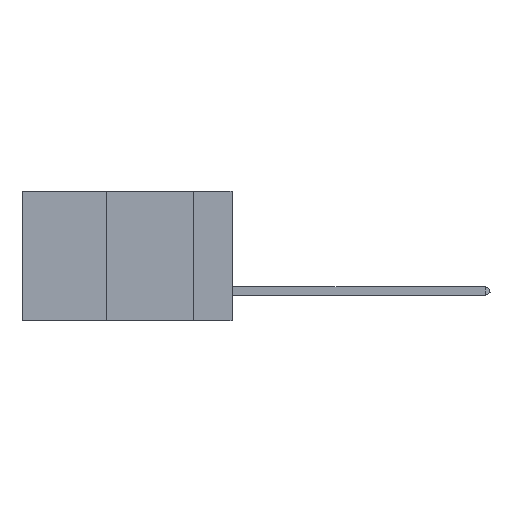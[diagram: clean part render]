
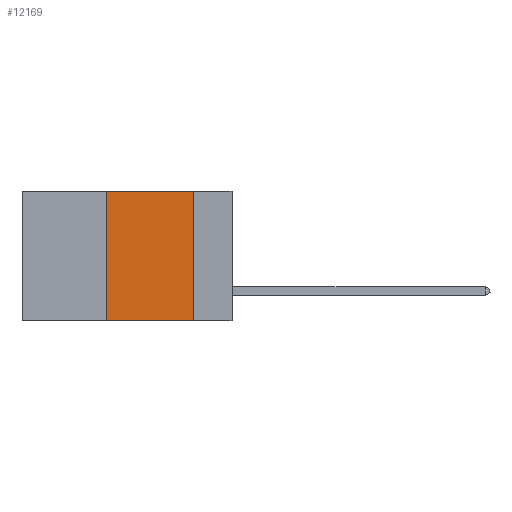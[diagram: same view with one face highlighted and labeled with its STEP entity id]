
A CAD part, left-side view. The second image highlights one B-rep face of the part: STEP entity #12169.
In plain terms, the highlighted planar face has unit normal (-1, 0, 0).
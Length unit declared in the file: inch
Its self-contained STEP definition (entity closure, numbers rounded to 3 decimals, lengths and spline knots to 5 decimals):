
#32 = CARTESIAN_POINT ( 'NONE',  ( 0., 0.11, 0. ) ) ;
#212 = CARTESIAN_POINT ( 'NONE',  ( 0., 0.11, -0.37 ) ) ;
#803 = EDGE_CURVE ( 'NONE', #2570, #10767, #3318, .T. ) ;
#1180 = PLANE ( 'NONE',  #1440 ) ;
#1357 = ORIENTED_EDGE ( 'NONE', *, *, #2284, .F. ) ;
#1440 = AXIS2_PLACEMENT_3D ( 'NONE', #4864, #9573, #8406 ) ;
#1543 = ORIENTED_EDGE ( 'NONE', *, *, #803, .T. ) ;
#2284 = EDGE_CURVE ( 'NONE', #2570, #11008, #9830, .T. ) ;
#2570 = VERTEX_POINT ( 'NONE', #6084 ) ;
#2836 = DIRECTION ( 'NONE',  ( 0., 0., -1. ) ) ;
#2902 = CARTESIAN_POINT ( 'NONE',  ( 0., 0.6, 0. ) ) ;
#2938 = VECTOR ( 'NONE', #14707, 39.37008 ) ;
#3318 = LINE ( 'NONE', #14278, #11174 ) ;
#4864 = CARTESIAN_POINT ( 'NONE',  ( 0., 0.6, 0. ) ) ;
#4875 = EDGE_CURVE ( 'NONE', #11008, #13784, #8199, .T. ) ;
#5167 = DIRECTION ( 'NONE',  ( 0., -1., 0. ) ) ;
#6084 = CARTESIAN_POINT ( 'NONE',  ( 0., 0.36, -0.37 ) ) ;
#6574 = LINE ( 'NONE', #9980, #13666 ) ;
#6877 = CARTESIAN_POINT ( 'NONE',  ( 0., 0.36, 0. ) ) ;
#7581 = ORIENTED_EDGE ( 'NONE', *, *, #8968, .F. ) ;
#8199 = LINE ( 'NONE', #2902, #12694 ) ;
#8406 = DIRECTION ( 'NONE',  ( 0., 0., -1. ) ) ;
#8968 = EDGE_CURVE ( 'NONE', #13784, #10767, #6574, .T. ) ;
#8987 = CARTESIAN_POINT ( 'NONE',  ( 0., 0.36, 0. ) ) ;
#9569 = ORIENTED_EDGE ( 'NONE', *, *, #4875, .F. ) ;
#9573 = DIRECTION ( 'NONE',  ( 1., 0., 0. ) ) ;
#9830 = LINE ( 'NONE', #8987, #2938 ) ;
#9980 = CARTESIAN_POINT ( 'NONE',  ( 0., 0.11, 0. ) ) ;
#10767 = VERTEX_POINT ( 'NONE', #212 ) ;
#11008 = VERTEX_POINT ( 'NONE', #6877 ) ;
#11174 = VECTOR ( 'NONE', #14375, 39.37008 ) ;
#12169 = ADVANCED_FACE ( 'NONE', ( #12757 ), #1180, .F. ) ;
#12694 = VECTOR ( 'NONE', #5167, 39.37008 ) ;
#12757 = FACE_OUTER_BOUND ( 'NONE', #14022, .T. ) ;
#13666 = VECTOR ( 'NONE', #2836, 39.37008 ) ;
#13784 = VERTEX_POINT ( 'NONE', #32 ) ;
#14022 = EDGE_LOOP ( 'NONE', ( #7581, #9569, #1357, #1543 ) ) ;
#14278 = CARTESIAN_POINT ( 'NONE',  ( 0., 0.6, -0.37 ) ) ;
#14375 = DIRECTION ( 'NONE',  ( 0., -1., 0. ) ) ;
#14707 = DIRECTION ( 'NONE',  ( 0., 0., 1. ) ) ;
